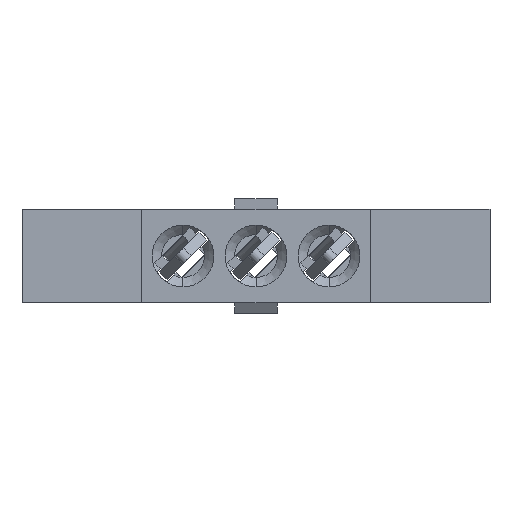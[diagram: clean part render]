
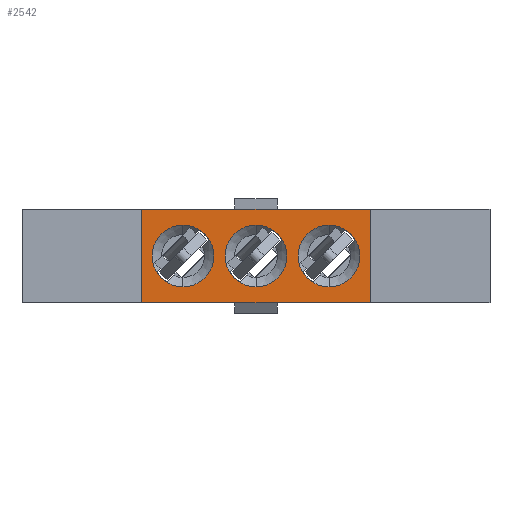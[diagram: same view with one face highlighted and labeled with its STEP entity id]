
A CAD part, front view. The second image highlights one B-rep face of the part: STEP entity #2542.
In plain terms, the highlighted planar face has unit normal (0, -1, 0).
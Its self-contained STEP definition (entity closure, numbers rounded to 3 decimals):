
#14 = ORIENTED_EDGE ( 'NONE', *, *, #6007, .T. ) ;
#75 = VERTEX_POINT ( 'NONE', #5359 ) ;
#133 = DIRECTION ( 'NONE',  ( 0., 1., 0. ) ) ;
#315 = ORIENTED_EDGE ( 'NONE', *, *, #523, .T. ) ;
#331 = AXIS2_PLACEMENT_3D ( 'NONE', #2243, #6436, #5857 ) ;
#463 = DIRECTION ( 'NONE',  ( 0., 0., 1. ) ) ;
#478 = EDGE_CURVE ( 'NONE', #3174, #2176, #4421, .T. ) ;
#505 = CARTESIAN_POINT ( 'NONE',  ( 10.16, -11.176, 2.54 ) ) ;
#523 = EDGE_CURVE ( 'NONE', #4861, #75, #4900, .T. ) ;
#605 = CARTESIAN_POINT ( 'NONE',  ( -2.235, -11.176, -2.54 ) ) ;
#607 = CARTESIAN_POINT ( 'NONE',  ( 7.925, -11.176, -1.676 ) ) ;
#700 = VECTOR ( 'NONE', #1451, 1000. ) ;
#928 = AXIS2_PLACEMENT_3D ( 'NONE', #4633, #4048, #4566 ) ;
#937 = CIRCLE ( 'NONE', #5330, 1.676 ) ;
#1126 = FACE_OUTER_BOUND ( 'NONE', #5346, .T. ) ;
#1234 = ORIENTED_EDGE ( 'NONE', *, *, #2382, .F. ) ;
#1451 = DIRECTION ( 'NONE',  ( 1., 0., 0. ) ) ;
#1467 = CIRCLE ( 'NONE', #6657, 1.676 ) ;
#1494 = DIRECTION ( 'NONE',  ( 0., 0., 1. ) ) ;
#1646 = CARTESIAN_POINT ( 'NONE',  ( 0., -11.176, 0. ) ) ;
#1656 = VECTOR ( 'NONE', #463, 1000. ) ;
#1705 = EDGE_CURVE ( 'NONE', #5069, #3927, #5802, .T. ) ;
#1798 = CARTESIAN_POINT ( 'NONE',  ( 0., -11.176, 0. ) ) ;
#1861 = CIRCLE ( 'NONE', #3898, 1.676 ) ;
#1975 = CARTESIAN_POINT ( 'NONE',  ( -2.235, -11.176, -2.54 ) ) ;
#2103 = DIRECTION ( 'NONE',  ( -1., 0., 0. ) ) ;
#2176 = VERTEX_POINT ( 'NONE', #3835 ) ;
#2243 = CARTESIAN_POINT ( 'NONE',  ( 0., -11.176, 0. ) ) ;
#2295 = VERTEX_POINT ( 'NONE', #6509 ) ;
#2382 = EDGE_CURVE ( 'NONE', #2176, #5069, #3038, .T. ) ;
#2456 = FACE_BOUND ( 'NONE', #6473, .T. ) ;
#2542 = ADVANCED_FACE ( 'NONE', ( #5049, #2882, #2456, #1126 ), #3305, .F. ) ;
#2740 = DIRECTION ( 'NONE',  ( 0., 1., 0. ) ) ;
#2764 = CARTESIAN_POINT ( 'NONE',  ( 7.925, -11.176, 0. ) ) ;
#2789 = LINE ( 'NONE', #6173, #700 ) ;
#2882 = FACE_BOUND ( 'NONE', #3968, .T. ) ;
#2986 = CARTESIAN_POINT ( 'NONE',  ( 10.16, -11.176, -2.54 ) ) ;
#3038 = LINE ( 'NONE', #605, #5631 ) ;
#3042 = DIRECTION ( 'NONE',  ( 0., 1., 0. ) ) ;
#3050 = DIRECTION ( 'NONE',  ( 0., 0., -1. ) ) ;
#3071 = EDGE_CURVE ( 'NONE', #4032, #6370, #937, .T. ) ;
#3144 = ORIENTED_EDGE ( 'NONE', *, *, #5159, .T. ) ;
#3174 = VERTEX_POINT ( 'NONE', #505 ) ;
#3280 = DIRECTION ( 'NONE',  ( 0., 0., 1. ) ) ;
#3305 = PLANE ( 'NONE',  #331 ) ;
#3464 = ORIENTED_EDGE ( 'NONE', *, *, #3071, .T. ) ;
#3835 = CARTESIAN_POINT ( 'NONE',  ( 10.16, -11.176, -2.54 ) ) ;
#3837 = EDGE_CURVE ( 'NONE', #75, #4861, #4731, .T. ) ;
#3898 = AXIS2_PLACEMENT_3D ( 'NONE', #1798, #6440, #4370 ) ;
#3927 = VERTEX_POINT ( 'NONE', #5647 ) ;
#3968 = EDGE_LOOP ( 'NONE', ( #315, #5945 ) ) ;
#4007 = CARTESIAN_POINT ( 'NONE',  ( 7.925, -11.176, 0. ) ) ;
#4032 = VERTEX_POINT ( 'NONE', #5183 ) ;
#4048 = DIRECTION ( 'NONE',  ( 0., 1., 0. ) ) ;
#4064 = DIRECTION ( 'NONE',  ( 0., 1., 0. ) ) ;
#4221 = ORIENTED_EDGE ( 'NONE', *, *, #1705, .F. ) ;
#4370 = DIRECTION ( 'NONE',  ( 0., 0., 1. ) ) ;
#4421 = LINE ( 'NONE', #2986, #6226 ) ;
#4498 = EDGE_CURVE ( 'NONE', #3927, #3174, #2789, .T. ) ;
#4510 = ORIENTED_EDGE ( 'NONE', *, *, #4498, .F. ) ;
#4566 = DIRECTION ( 'NONE',  ( 0., 0., 1. ) ) ;
#4633 = CARTESIAN_POINT ( 'NONE',  ( 3.962, -11.176, 0. ) ) ;
#4709 = CARTESIAN_POINT ( 'NONE',  ( 3.962, -11.176, 1.676 ) ) ;
#4731 = CIRCLE ( 'NONE', #4847, 1.676 ) ;
#4847 = AXIS2_PLACEMENT_3D ( 'NONE', #6113, #3042, #6701 ) ;
#4861 = VERTEX_POINT ( 'NONE', #4709 ) ;
#4900 = CIRCLE ( 'NONE', #928, 1.676 ) ;
#5049 = FACE_BOUND ( 'NONE', #6704, .T. ) ;
#5069 = VERTEX_POINT ( 'NONE', #6357 ) ;
#5159 = EDGE_CURVE ( 'NONE', #6590, #2295, #1861, .T. ) ;
#5183 = CARTESIAN_POINT ( 'NONE',  ( 7.925, -11.176, 1.676 ) ) ;
#5330 = AXIS2_PLACEMENT_3D ( 'NONE', #2764, #2740, #3280 ) ;
#5346 = EDGE_LOOP ( 'NONE', ( #4221, #1234, #6033, #4510 ) ) ;
#5359 = CARTESIAN_POINT ( 'NONE',  ( 3.962, -11.176, -1.676 ) ) ;
#5523 = EDGE_CURVE ( 'NONE', #2295, #6590, #5868, .T. ) ;
#5631 = VECTOR ( 'NONE', #2103, 1000. ) ;
#5647 = CARTESIAN_POINT ( 'NONE',  ( -2.235, -11.176, 2.54 ) ) ;
#5700 = DIRECTION ( 'NONE',  ( 0., 0., 1. ) ) ;
#5802 = LINE ( 'NONE', #1975, #1656 ) ;
#5857 = DIRECTION ( 'NONE',  ( 0., 0., 1. ) ) ;
#5868 = CIRCLE ( 'NONE', #6108, 1.676 ) ;
#5910 = ORIENTED_EDGE ( 'NONE', *, *, #5523, .T. ) ;
#5945 = ORIENTED_EDGE ( 'NONE', *, *, #3837, .T. ) ;
#6007 = EDGE_CURVE ( 'NONE', #6370, #4032, #1467, .T. ) ;
#6033 = ORIENTED_EDGE ( 'NONE', *, *, #478, .F. ) ;
#6061 = CARTESIAN_POINT ( 'NONE',  ( 0., -11.176, -1.676 ) ) ;
#6108 = AXIS2_PLACEMENT_3D ( 'NONE', #1646, #133, #5700 ) ;
#6113 = CARTESIAN_POINT ( 'NONE',  ( 3.962, -11.176, 0. ) ) ;
#6173 = CARTESIAN_POINT ( 'NONE',  ( -2.235, -11.176, 2.54 ) ) ;
#6226 = VECTOR ( 'NONE', #3050, 1000. ) ;
#6357 = CARTESIAN_POINT ( 'NONE',  ( -2.235, -11.176, -2.54 ) ) ;
#6370 = VERTEX_POINT ( 'NONE', #607 ) ;
#6436 = DIRECTION ( 'NONE',  ( 0., 1., 0. ) ) ;
#6440 = DIRECTION ( 'NONE',  ( 0., 1., 0. ) ) ;
#6473 = EDGE_LOOP ( 'NONE', ( #5910, #3144 ) ) ;
#6509 = CARTESIAN_POINT ( 'NONE',  ( 0., -11.176, 1.676 ) ) ;
#6590 = VERTEX_POINT ( 'NONE', #6061 ) ;
#6657 = AXIS2_PLACEMENT_3D ( 'NONE', #4007, #4064, #1494 ) ;
#6701 = DIRECTION ( 'NONE',  ( 0., 0., 1. ) ) ;
#6704 = EDGE_LOOP ( 'NONE', ( #3464, #14 ) ) ;
